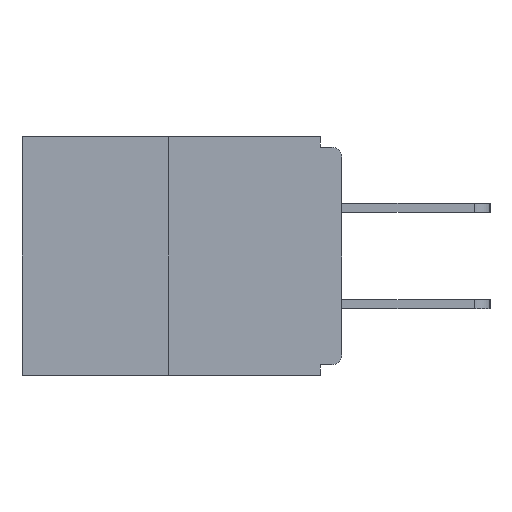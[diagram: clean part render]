
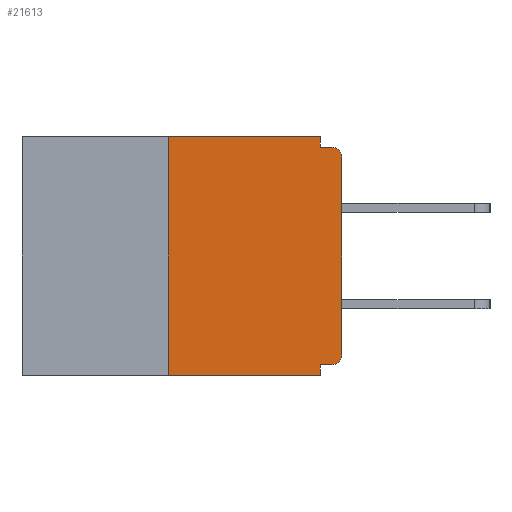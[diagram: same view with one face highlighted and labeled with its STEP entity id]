
A CAD part, left-side view. The second image highlights one B-rep face of the part: STEP entity #21613.
In plain terms, the highlighted planar face has unit normal (-1, 0, 0).
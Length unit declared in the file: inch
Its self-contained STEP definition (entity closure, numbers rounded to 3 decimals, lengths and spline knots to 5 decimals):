
#754 = CARTESIAN_POINT ( 'NONE',  ( 0., 0.015, -0.328 ) ) ;
#918 = VECTOR ( 'NONE', #13954, 39.37008 ) ;
#1019 = VERTEX_POINT ( 'NONE', #21411 ) ;
#1143 = CARTESIAN_POINT ( 'NONE',  ( 0., 0.031, 0. ) ) ;
#1993 = PLANE ( 'NONE',  #6827 ) ;
#2073 = DIRECTION ( 'NONE',  ( 1., 0., 0. ) ) ;
#2265 = AXIS2_PLACEMENT_3D ( 'NONE', #12292, #22217, #20337 ) ;
#2939 = ORIENTED_EDGE ( 'NONE', *, *, #17203, .T. ) ;
#3016 = LINE ( 'NONE', #17389, #22089 ) ;
#3141 = CIRCLE ( 'NONE', #2265, 0.015 ) ;
#3219 = EDGE_CURVE ( 'NONE', #17753, #13631, #16183, .T. ) ;
#3880 = AXIS2_PLACEMENT_3D ( 'NONE', #9077, #25192, #4746 ) ;
#4145 = ORIENTED_EDGE ( 'NONE', *, *, #17816, .T. ) ;
#4416 = LINE ( 'NONE', #24537, #918 ) ;
#4672 = VERTEX_POINT ( 'NONE', #754 ) ;
#4746 = DIRECTION ( 'NONE',  ( 0., 0., -1. ) ) ;
#5638 = EDGE_CURVE ( 'NONE', #4672, #25093, #3016, .T. ) ;
#6332 = CARTESIAN_POINT ( 'NONE',  ( 0., 0.031, 0. ) ) ;
#6658 = CARTESIAN_POINT ( 'NONE',  ( 0., 0., -0.03 ) ) ;
#6699 = VECTOR ( 'NONE', #16189, 39.37008 ) ;
#6827 = AXIS2_PLACEMENT_3D ( 'NONE', #14247, #2073, #8024 ) ;
#7271 = DIRECTION ( 'NONE',  ( 0., 1., 0. ) ) ;
#7715 = CARTESIAN_POINT ( 'NONE',  ( 0., 0.25, 0. ) ) ;
#8024 = DIRECTION ( 'NONE',  ( 0., 0., -1. ) ) ;
#8120 = EDGE_CURVE ( 'NONE', #25684, #10383, #25953, .T. ) ;
#8592 = DIRECTION ( 'NONE',  ( 0., 0., 1. ) ) ;
#8594 = VERTEX_POINT ( 'NONE', #22484 ) ;
#9077 = CARTESIAN_POINT ( 'NONE',  ( 0., 0.015, -0.313 ) ) ;
#9745 = VERTEX_POINT ( 'NONE', #6658 ) ;
#9773 = VERTEX_POINT ( 'NONE', #20879 ) ;
#9802 = CARTESIAN_POINT ( 'NONE',  ( 0., 0., -0.015 ) ) ;
#9831 = ORIENTED_EDGE ( 'NONE', *, *, #10458, .F. ) ;
#10383 = VERTEX_POINT ( 'NONE', #25911 ) ;
#10458 = EDGE_CURVE ( 'NONE', #10383, #1019, #17515, .T. ) ;
#10842 = EDGE_CURVE ( 'NONE', #25093, #8594, #20035, .T. ) ;
#11157 = CARTESIAN_POINT ( 'NONE',  ( 0., 0.25, 0. ) ) ;
#11228 = CARTESIAN_POINT ( 'NONE',  ( 0., 0.031, -0.343 ) ) ;
#11419 = DIRECTION ( 'NONE',  ( 0., 0., 1. ) ) ;
#11544 = EDGE_CURVE ( 'NONE', #13631, #25684, #4416, .T. ) ;
#11549 = EDGE_CURVE ( 'NONE', #9745, #1019, #3141, .T. ) ;
#12292 = CARTESIAN_POINT ( 'NONE',  ( 0., 0.015, -0.03 ) ) ;
#13200 = CIRCLE ( 'NONE', #3880, 0.015 ) ;
#13631 = VERTEX_POINT ( 'NONE', #7715 ) ;
#13954 = DIRECTION ( 'NONE',  ( 0., -1., 0. ) ) ;
#14247 = CARTESIAN_POINT ( 'NONE',  ( 0., 0.46, 0. ) ) ;
#14902 = VECTOR ( 'NONE', #11419, 39.37008 ) ;
#15373 = FACE_OUTER_BOUND ( 'NONE', #18276, .T. ) ;
#15384 = LINE ( 'NONE', #18715, #16032 ) ;
#15388 = ORIENTED_EDGE ( 'NONE', *, *, #15713, .T. ) ;
#15613 = CARTESIAN_POINT ( 'NONE',  ( 0., 0.25, -0.343 ) ) ;
#15713 = EDGE_CURVE ( 'NONE', #9773, #9745, #15384, .T. ) ;
#16032 = VECTOR ( 'NONE', #8592, 39.37008 ) ;
#16183 = LINE ( 'NONE', #11157, #14902 ) ;
#16189 = DIRECTION ( 'NONE',  ( 0., -1., 0. ) ) ;
#16290 = ORIENTED_EDGE ( 'NONE', *, *, #8120, .F. ) ;
#17108 = ORIENTED_EDGE ( 'NONE', *, *, #3219, .F. ) ;
#17184 = VECTOR ( 'NONE', #19175, 39.37008 ) ;
#17203 = EDGE_CURVE ( 'NONE', #4672, #9773, #13200, .T. ) ;
#17389 = CARTESIAN_POINT ( 'NONE',  ( 0., 0., -0.328 ) ) ;
#17515 = LINE ( 'NONE', #9802, #6699 ) ;
#17517 = CARTESIAN_POINT ( 'NONE',  ( 0., 0.031, -0.328 ) ) ;
#17753 = VERTEX_POINT ( 'NONE', #15613 ) ;
#17816 = EDGE_CURVE ( 'NONE', #17753, #8594, #23521, .T. ) ;
#18276 = EDGE_LOOP ( 'NONE', ( #24767, #17108, #4145, #22946, #22907, #2939, #15388, #18622, #9831, #16290 ) ) ;
#18622 = ORIENTED_EDGE ( 'NONE', *, *, #11549, .T. ) ;
#18715 = CARTESIAN_POINT ( 'NONE',  ( 0., 0., 0. ) ) ;
#19175 = DIRECTION ( 'NONE',  ( 0., 0., -1. ) ) ;
#20035 = LINE ( 'NONE', #11228, #17184 ) ;
#20174 = DIRECTION ( 'NONE',  ( 0., -1., 0. ) ) ;
#20191 = VECTOR ( 'NONE', #21395, 39.37008 ) ;
#20337 = DIRECTION ( 'NONE',  ( 0., 0., -1. ) ) ;
#20879 = CARTESIAN_POINT ( 'NONE',  ( 0., 0., -0.313 ) ) ;
#21395 = DIRECTION ( 'NONE',  ( 0., 0., -1. ) ) ;
#21411 = CARTESIAN_POINT ( 'NONE',  ( 0., 0.015, -0.015 ) ) ;
#21613 = ADVANCED_FACE ( 'NONE', ( #15373 ), #1993, .F. ) ;
#22089 = VECTOR ( 'NONE', #7271, 39.37008 ) ;
#22217 = DIRECTION ( 'NONE',  ( -1., 0., 0. ) ) ;
#22270 = CARTESIAN_POINT ( 'NONE',  ( 0., 0.46, -0.343 ) ) ;
#22484 = CARTESIAN_POINT ( 'NONE',  ( 0., 0.031, -0.343 ) ) ;
#22907 = ORIENTED_EDGE ( 'NONE', *, *, #5638, .F. ) ;
#22946 = ORIENTED_EDGE ( 'NONE', *, *, #10842, .F. ) ;
#23521 = LINE ( 'NONE', #22270, #24163 ) ;
#24163 = VECTOR ( 'NONE', #20174, 39.37008 ) ;
#24537 = CARTESIAN_POINT ( 'NONE',  ( 0., 0.46, 0. ) ) ;
#24767 = ORIENTED_EDGE ( 'NONE', *, *, #11544, .F. ) ;
#25093 = VERTEX_POINT ( 'NONE', #17517 ) ;
#25192 = DIRECTION ( 'NONE',  ( -1., 0., 0. ) ) ;
#25684 = VERTEX_POINT ( 'NONE', #6332 ) ;
#25911 = CARTESIAN_POINT ( 'NONE',  ( 0., 0.031, -0.015 ) ) ;
#25953 = LINE ( 'NONE', #1143, #20191 ) ;
